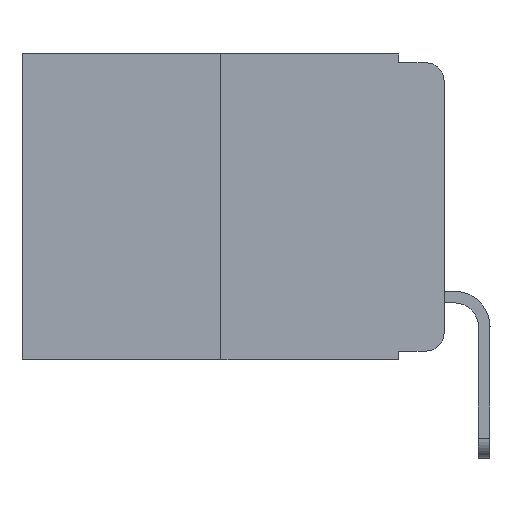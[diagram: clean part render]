
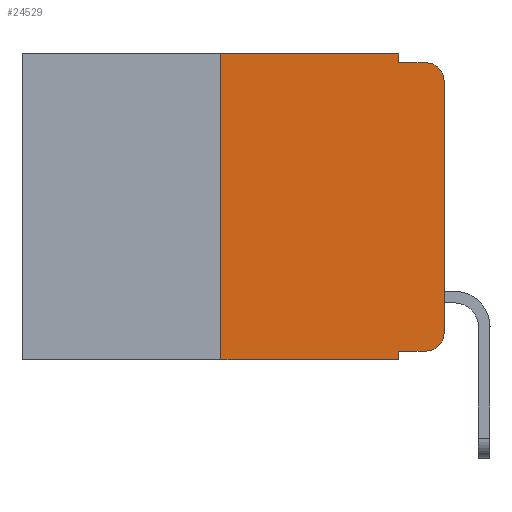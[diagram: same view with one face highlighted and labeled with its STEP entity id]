
A CAD part, left-side view. The second image highlights one B-rep face of the part: STEP entity #24529.
In plain terms, the highlighted planar face has unit normal (-1, 0, 0).
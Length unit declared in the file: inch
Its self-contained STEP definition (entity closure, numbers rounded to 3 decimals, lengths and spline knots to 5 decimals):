
#248 = CARTESIAN_POINT ( 'NONE',  ( 0., 0.473, 0. ) ) ;
#355 = CARTESIAN_POINT ( 'NONE',  ( 0., 0.051, -0.01 ) ) ;
#869 = EDGE_CURVE ( 'NONE', #10596, #12832, #7457, .T. ) ;
#920 = CARTESIAN_POINT ( 'NONE',  ( 0., 0., -0.03 ) ) ;
#2321 = CARTESIAN_POINT ( 'NONE',  ( 0., 0.25, -0.343 ) ) ;
#2390 = DIRECTION ( 'NONE',  ( -1., 0., 0. ) ) ;
#3220 = CARTESIAN_POINT ( 'NONE',  ( 0., 0.051, -0.333 ) ) ;
#3604 = CARTESIAN_POINT ( 'NONE',  ( 0., 0.051, 0. ) ) ;
#3817 = CARTESIAN_POINT ( 'NONE',  ( 0., 0.051, -0.343 ) ) ;
#4286 = ORIENTED_EDGE ( 'NONE', *, *, #16909, .T. ) ;
#4544 = ORIENTED_EDGE ( 'NONE', *, *, #7816, .F. ) ;
#4800 = CARTESIAN_POINT ( 'NONE',  ( 0., 0.02, -0.313 ) ) ;
#5152 = VECTOR ( 'NONE', #17161, 39.37008 ) ;
#5178 = CARTESIAN_POINT ( 'NONE',  ( 0., 0.051, 0. ) ) ;
#5311 = VERTEX_POINT ( 'NONE', #20356 ) ;
#5532 = LINE ( 'NONE', #24783, #20228 ) ;
#5917 = VERTEX_POINT ( 'NONE', #3604 ) ;
#6720 = FACE_OUTER_BOUND ( 'NONE', #22867, .T. ) ;
#6900 = ORIENTED_EDGE ( 'NONE', *, *, #10358, .F. ) ;
#7405 = VERTEX_POINT ( 'NONE', #10859 ) ;
#7457 = LINE ( 'NONE', #16910, #5152 ) ;
#7811 = AXIS2_PLACEMENT_3D ( 'NONE', #15973, #2390, #12419 ) ;
#7816 = EDGE_CURVE ( 'NONE', #5917, #5311, #19321, .T. ) ;
#7911 = VERTEX_POINT ( 'NONE', #12027 ) ;
#8976 = AXIS2_PLACEMENT_3D ( 'NONE', #4800, #20140, #10577 ) ;
#9120 = ORIENTED_EDGE ( 'NONE', *, *, #9166, .F. ) ;
#9166 = EDGE_CURVE ( 'NONE', #5311, #7911, #17579, .T. ) ;
#9339 = EDGE_CURVE ( 'NONE', #10411, #7405, #20440, .T. ) ;
#9722 = CARTESIAN_POINT ( 'NONE',  ( 0., 0.473, -0.343 ) ) ;
#9763 = DIRECTION ( 'NONE',  ( 0., 0., -1. ) ) ;
#9853 = AXIS2_PLACEMENT_3D ( 'NONE', #22065, #13158, #11515 ) ;
#10358 = EDGE_CURVE ( 'NONE', #22656, #15339, #5532, .T. ) ;
#10411 = VERTEX_POINT ( 'NONE', #13336 ) ;
#10523 = VECTOR ( 'NONE', #12901, 39.37008 ) ;
#10577 = DIRECTION ( 'NONE',  ( 0., 0., -1. ) ) ;
#10596 = VERTEX_POINT ( 'NONE', #23240 ) ;
#10859 = CARTESIAN_POINT ( 'NONE',  ( 0., 0.02, -0.333 ) ) ;
#11247 = VERTEX_POINT ( 'NONE', #3817 ) ;
#11259 = VECTOR ( 'NONE', #20778, 39.37008 ) ;
#11493 = DIRECTION ( 'NONE',  ( 0., -1., 0. ) ) ;
#11515 = DIRECTION ( 'NONE',  ( 0., 0., -1. ) ) ;
#12027 = CARTESIAN_POINT ( 'NONE',  ( 0., 0.02, -0.01 ) ) ;
#12180 = ORIENTED_EDGE ( 'NONE', *, *, #23862, .T. ) ;
#12419 = DIRECTION ( 'NONE',  ( 0., 0., -1. ) ) ;
#12832 = VERTEX_POINT ( 'NONE', #920 ) ;
#12901 = DIRECTION ( 'NONE',  ( 0., -1., 0. ) ) ;
#13158 = DIRECTION ( 'NONE',  ( 1., 0., 0. ) ) ;
#13336 = CARTESIAN_POINT ( 'NONE',  ( 0., 0.051, -0.333 ) ) ;
#14397 = PLANE ( 'NONE',  #9853 ) ;
#14703 = ORIENTED_EDGE ( 'NONE', *, *, #869, .T. ) ;
#14875 = VECTOR ( 'NONE', #16078, 39.37008 ) ;
#15319 = ORIENTED_EDGE ( 'NONE', *, *, #22883, .T. ) ;
#15339 = VERTEX_POINT ( 'NONE', #20449 ) ;
#15454 = CIRCLE ( 'NONE', #7811, 0.02 ) ;
#15588 = LINE ( 'NONE', #248, #14875 ) ;
#15973 = CARTESIAN_POINT ( 'NONE',  ( 0., 0.02, -0.03 ) ) ;
#16078 = DIRECTION ( 'NONE',  ( 0., -1., 0. ) ) ;
#16581 = VECTOR ( 'NONE', #22377, 39.37008 ) ;
#16909 = EDGE_CURVE ( 'NONE', #22656, #11247, #19048, .T. ) ;
#16910 = CARTESIAN_POINT ( 'NONE',  ( 0., 0., 0. ) ) ;
#17118 = DIRECTION ( 'NONE',  ( 0., 0., 1. ) ) ;
#17161 = DIRECTION ( 'NONE',  ( 0., 0., 1. ) ) ;
#17579 = LINE ( 'NONE', #355, #16581 ) ;
#17817 = CIRCLE ( 'NONE', #8976, 0.02 ) ;
#17954 = EDGE_CURVE ( 'NONE', #15339, #5917, #15588, .T. ) ;
#18465 = EDGE_CURVE ( 'NONE', #10411, #11247, #22146, .T. ) ;
#19048 = LINE ( 'NONE', #9722, #22455 ) ;
#19090 = CARTESIAN_POINT ( 'NONE',  ( 0., 0.051, 0. ) ) ;
#19321 = LINE ( 'NONE', #19090, #22572 ) ;
#19615 = ORIENTED_EDGE ( 'NONE', *, *, #18465, .F. ) ;
#20061 = ORIENTED_EDGE ( 'NONE', *, *, #9339, .T. ) ;
#20140 = DIRECTION ( 'NONE',  ( -1., 0., 0. ) ) ;
#20228 = VECTOR ( 'NONE', #17118, 39.37008 ) ;
#20356 = CARTESIAN_POINT ( 'NONE',  ( 0., 0.051, -0.01 ) ) ;
#20440 = LINE ( 'NONE', #3220, #10523 ) ;
#20449 = CARTESIAN_POINT ( 'NONE',  ( 0., 0.25, 0. ) ) ;
#20778 = DIRECTION ( 'NONE',  ( 0., 0., -1. ) ) ;
#22065 = CARTESIAN_POINT ( 'NONE',  ( 0., 0.473, 0. ) ) ;
#22146 = LINE ( 'NONE', #5178, #11259 ) ;
#22377 = DIRECTION ( 'NONE',  ( 0., -1., 0. ) ) ;
#22455 = VECTOR ( 'NONE', #11493, 39.37008 ) ;
#22572 = VECTOR ( 'NONE', #9763, 39.37008 ) ;
#22656 = VERTEX_POINT ( 'NONE', #2321 ) ;
#22867 = EDGE_LOOP ( 'NONE', ( #14703, #12180, #9120, #4544, #24125, #6900, #4286, #19615, #20061, #15319 ) ) ;
#22883 = EDGE_CURVE ( 'NONE', #7405, #10596, #17817, .T. ) ;
#23240 = CARTESIAN_POINT ( 'NONE',  ( 0., 0., -0.313 ) ) ;
#23862 = EDGE_CURVE ( 'NONE', #12832, #7911, #15454, .T. ) ;
#24125 = ORIENTED_EDGE ( 'NONE', *, *, #17954, .F. ) ;
#24529 = ADVANCED_FACE ( 'NONE', ( #6720 ), #14397, .F. ) ;
#24783 = CARTESIAN_POINT ( 'NONE',  ( 0., 0.25, 0. ) ) ;
